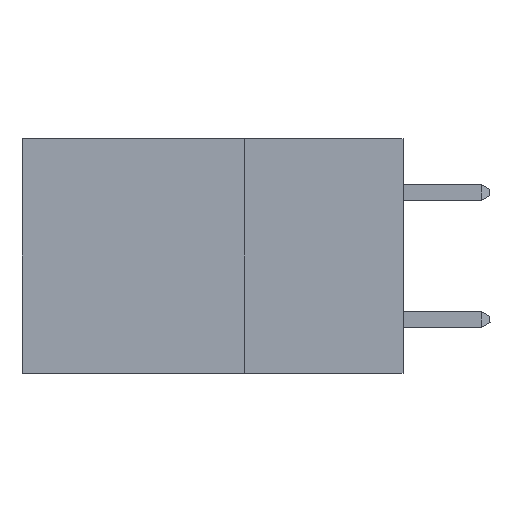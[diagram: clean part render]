
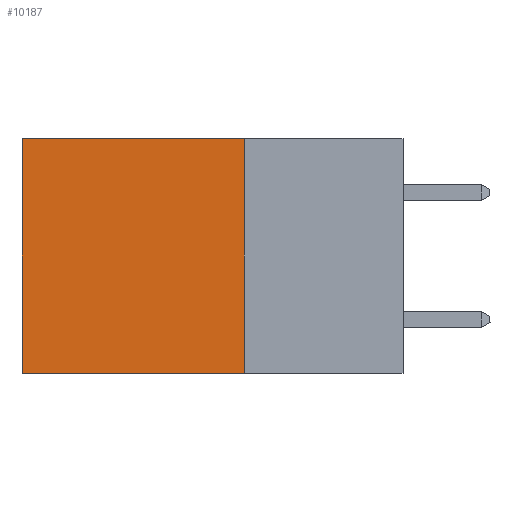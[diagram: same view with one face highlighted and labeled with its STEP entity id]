
A CAD part, left-side view. The second image highlights one B-rep face of the part: STEP entity #10187.
In plain terms, the highlighted planar face has unit normal (-1, 0, 0).
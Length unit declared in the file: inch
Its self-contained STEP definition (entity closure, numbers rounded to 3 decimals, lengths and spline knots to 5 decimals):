
#930 = AXIS2_PLACEMENT_3D ( 'NONE', #23180, #8662, #27914 ) ;
#1726 = EDGE_CURVE ( 'NONE', #19956, #19202, #1751, .T. ) ;
#1751 = LINE ( 'NONE', #23033, #20064 ) ;
#1864 = DIRECTION ( 'NONE',  ( 0., 0., -1. ) ) ;
#2430 = LINE ( 'NONE', #26401, #12496 ) ;
#3029 = ORIENTED_EDGE ( 'NONE', *, *, #26369, .T. ) ;
#3030 = LINE ( 'NONE', #21234, #17212 ) ;
#6301 = PLANE ( 'NONE',  #930 ) ;
#6568 = CARTESIAN_POINT ( 'NONE',  ( 0.2875, 0.6, 0. ) ) ;
#7657 = ORIENTED_EDGE ( 'NONE', *, *, #1726, .F. ) ;
#8662 = DIRECTION ( 'NONE',  ( 1., 0., 0. ) ) ;
#8946 = DIRECTION ( 'NONE',  ( 0., 1., 0. ) ) ;
#10187 = ADVANCED_FACE ( 'NONE', ( #15167 ), #6301, .F. ) ;
#10500 = VERTEX_POINT ( 'NONE', #21523 ) ;
#11039 = DIRECTION ( 'NONE',  ( 0., 0., -1. ) ) ;
#11063 = ORIENTED_EDGE ( 'NONE', *, *, #16181, .F. ) ;
#12496 = VECTOR ( 'NONE', #19127, 39.37008 ) ;
#15167 = FACE_OUTER_BOUND ( 'NONE', #30036, .T. ) ;
#16181 = EDGE_CURVE ( 'NONE', #19202, #10500, #3030, .T. ) ;
#17212 = VECTOR ( 'NONE', #8946, 39.37008 ) ;
#19127 = DIRECTION ( 'NONE',  ( 0., 1., 0. ) ) ;
#19202 = VERTEX_POINT ( 'NONE', #28035 ) ;
#19918 = VERTEX_POINT ( 'NONE', #28193 ) ;
#19956 = VERTEX_POINT ( 'NONE', #21025 ) ;
#20049 = ORIENTED_EDGE ( 'NONE', *, *, #28002, .T. ) ;
#20064 = VECTOR ( 'NONE', #11039, 39.37008 ) ;
#21025 = CARTESIAN_POINT ( 'NONE',  ( 0.2875, 0.25, 0. ) ) ;
#21234 = CARTESIAN_POINT ( 'NONE',  ( 0.2875, 0.25, -0.37 ) ) ;
#21523 = CARTESIAN_POINT ( 'NONE',  ( 0.2875, 0.6, -0.37 ) ) ;
#23033 = CARTESIAN_POINT ( 'NONE',  ( 0.2875, 0.25, 0. ) ) ;
#23180 = CARTESIAN_POINT ( 'NONE',  ( 0.2875, 0.25, 0. ) ) ;
#26369 = EDGE_CURVE ( 'NONE', #19956, #19918, #2430, .T. ) ;
#26401 = CARTESIAN_POINT ( 'NONE',  ( 0.2875, 0.25, 0. ) ) ;
#27914 = DIRECTION ( 'NONE',  ( 0., 0., -1. ) ) ;
#28002 = EDGE_CURVE ( 'NONE', #19918, #10500, #30898, .T. ) ;
#28035 = CARTESIAN_POINT ( 'NONE',  ( 0.2875, 0.25, -0.37 ) ) ;
#28193 = CARTESIAN_POINT ( 'NONE',  ( 0.2875, 0.6, 0. ) ) ;
#28972 = VECTOR ( 'NONE', #1864, 39.37008 ) ;
#30036 = EDGE_LOOP ( 'NONE', ( #20049, #11063, #7657, #3029 ) ) ;
#30898 = LINE ( 'NONE', #6568, #28972 ) ;
